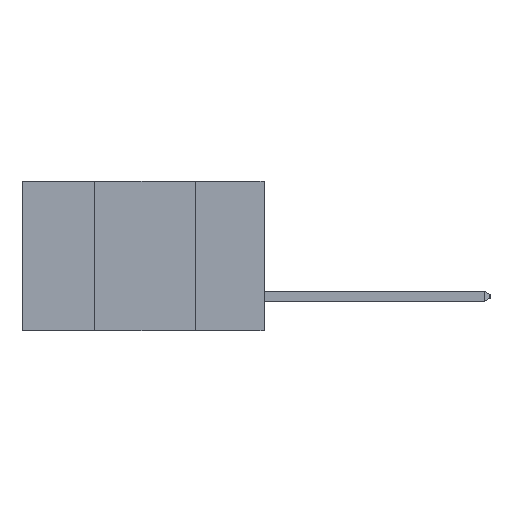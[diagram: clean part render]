
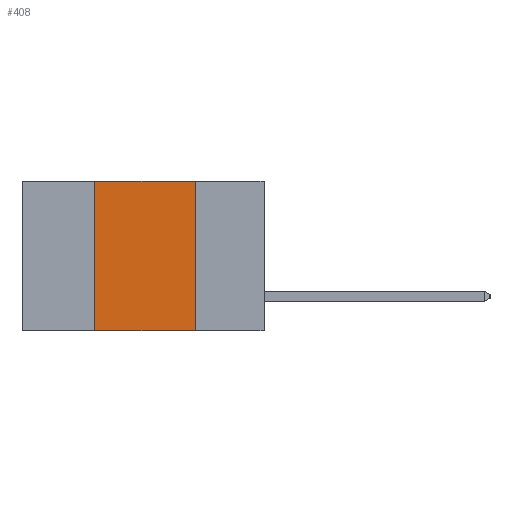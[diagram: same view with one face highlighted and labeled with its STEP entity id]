
A CAD part, left-side view. The second image highlights one B-rep face of the part: STEP entity #408.
In plain terms, the highlighted planar face has unit normal (-1, 0, 0).
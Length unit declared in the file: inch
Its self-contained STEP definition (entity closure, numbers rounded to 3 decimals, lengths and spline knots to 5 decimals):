
#408 = ADVANCED_FACE ( 'NONE', ( #3505 ), #5475, .F. ) ;
#552 = ORIENTED_EDGE ( 'NONE', *, *, #13040, .F. ) ;
#670 = DIRECTION ( 'NONE',  ( 0., -1., 0. ) ) ;
#933 = VERTEX_POINT ( 'NONE', #1713 ) ;
#1314 = VERTEX_POINT ( 'NONE', #15067 ) ;
#1713 = CARTESIAN_POINT ( 'NONE',  ( 0., 0.17, -0.37 ) ) ;
#2134 = CARTESIAN_POINT ( 'NONE',  ( 0., 0.42, 0. ) ) ;
#2278 = CARTESIAN_POINT ( 'NONE',  ( 0., 0.6, 0. ) ) ;
#3216 = EDGE_CURVE ( 'NONE', #3272, #933, #4240, .T. ) ;
#3272 = VERTEX_POINT ( 'NONE', #13810 ) ;
#3505 = FACE_OUTER_BOUND ( 'NONE', #8145, .T. ) ;
#3548 = VECTOR ( 'NONE', #4143, 39.37008 ) ;
#3974 = ORIENTED_EDGE ( 'NONE', *, *, #9344, .T. ) ;
#4143 = DIRECTION ( 'NONE',  ( 0., 0., 1. ) ) ;
#4240 = LINE ( 'NONE', #5989, #10245 ) ;
#5475 = PLANE ( 'NONE',  #13616 ) ;
#5989 = CARTESIAN_POINT ( 'NONE',  ( 0., 0.17, 0. ) ) ;
#7361 = LINE ( 'NONE', #14909, #9783 ) ;
#8145 = EDGE_LOOP ( 'NONE', ( #13396, #552, #11079, #3974 ) ) ;
#8562 = VECTOR ( 'NONE', #12407, 39.37008 ) ;
#8801 = LINE ( 'NONE', #10122, #3548 ) ;
#9344 = EDGE_CURVE ( 'NONE', #1314, #933, #7361, .T. ) ;
#9783 = VECTOR ( 'NONE', #670, 39.37008 ) ;
#9838 = DIRECTION ( 'NONE',  ( 1., 0., 0. ) ) ;
#9854 = DIRECTION ( 'NONE',  ( 0., 0., -1. ) ) ;
#10122 = CARTESIAN_POINT ( 'NONE',  ( 0., 0.42, 0. ) ) ;
#10245 = VECTOR ( 'NONE', #14665, 39.37008 ) ;
#10434 = EDGE_CURVE ( 'NONE', #1314, #13304, #8801, .T. ) ;
#11079 = ORIENTED_EDGE ( 'NONE', *, *, #10434, .F. ) ;
#11235 = CARTESIAN_POINT ( 'NONE',  ( 0., 0.6, 0. ) ) ;
#11346 = LINE ( 'NONE', #11235, #8562 ) ;
#12407 = DIRECTION ( 'NONE',  ( 0., -1., 0. ) ) ;
#13040 = EDGE_CURVE ( 'NONE', #13304, #3272, #11346, .T. ) ;
#13304 = VERTEX_POINT ( 'NONE', #2134 ) ;
#13396 = ORIENTED_EDGE ( 'NONE', *, *, #3216, .F. ) ;
#13616 = AXIS2_PLACEMENT_3D ( 'NONE', #2278, #9838, #9854 ) ;
#13810 = CARTESIAN_POINT ( 'NONE',  ( 0., 0.17, 0. ) ) ;
#14665 = DIRECTION ( 'NONE',  ( 0., 0., -1. ) ) ;
#14909 = CARTESIAN_POINT ( 'NONE',  ( 0., 0.6, -0.37 ) ) ;
#15067 = CARTESIAN_POINT ( 'NONE',  ( 0., 0.42, -0.37 ) ) ;
